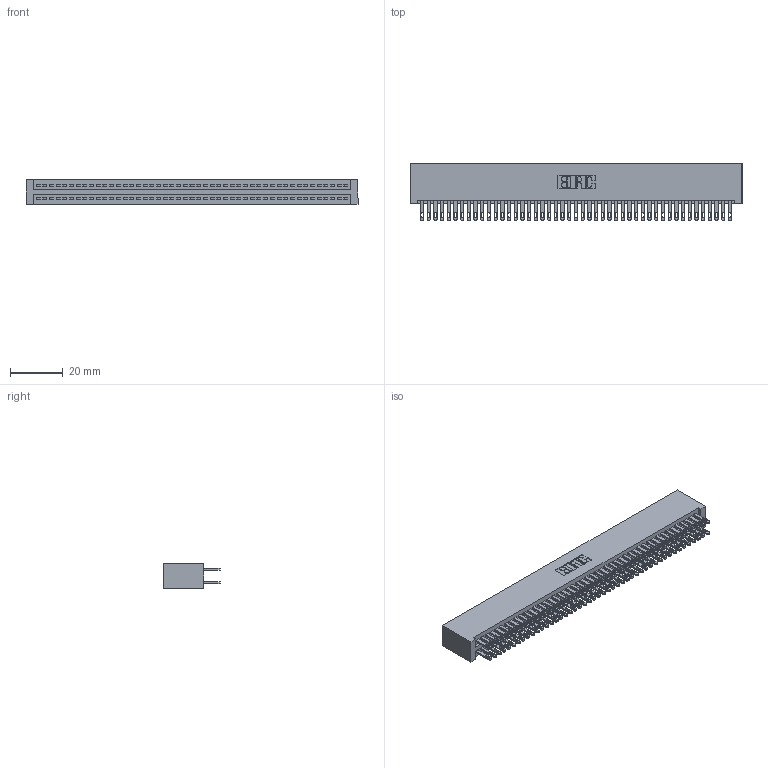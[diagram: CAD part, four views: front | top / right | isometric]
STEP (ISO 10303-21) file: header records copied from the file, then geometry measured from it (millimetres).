
FILE_DESCRIPTION (( 'STEP AP203' ), '1' );
FILE_NAME ('345-094-500-201.STEP', '2018-10-04T23:03:46', ( '' ), ( '' ), 'SwSTEP 2.0', 'SolidWorks 2016', '' );
FILE_SCHEMA (( 'CONFIG_CONTROL_DESIGN' ));
Length unit declared in the file: inch
Products named in the file (3): 345 Part_No Mounting Lugs; 345-094-500-201; 345-292-001_345-293-100
Assembly tree (95 placements, depth 2):
  345-094-500-201
    345 Part_No Mounting Lugs
    345-292-001_345-293-100  x94
Bounding box: 125.98 x 21.51 x 9.4 mm (x, y, z)
Volume: 13187.8 mm3; surface area: 20852.6 mm2
Topology: 95 solids, 95 shells, 4442 faces, 13571 edges, 9046 vertices
Faces by surface type: plane 2614, cylinder 1828
Entity records: 35857 total; most frequent: CARTESIAN_POINT 6004, ORIENTED_EDGE 5938, DIRECTION 5285, EDGE_CURVE 2969, VECTOR 2653, LINE 2653, VERTEX_POINT 1978, AXIS2_PLACEMENT_3D 1316
